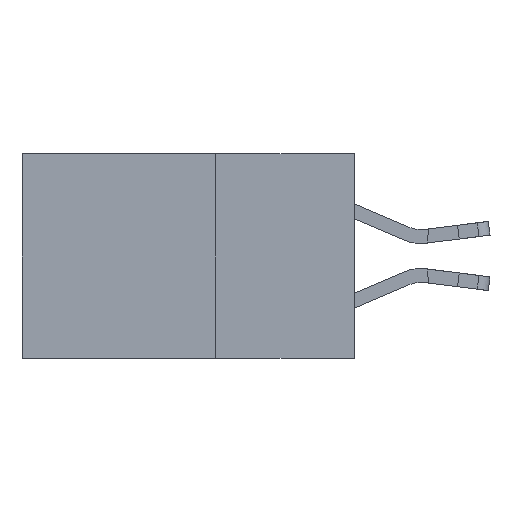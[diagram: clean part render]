
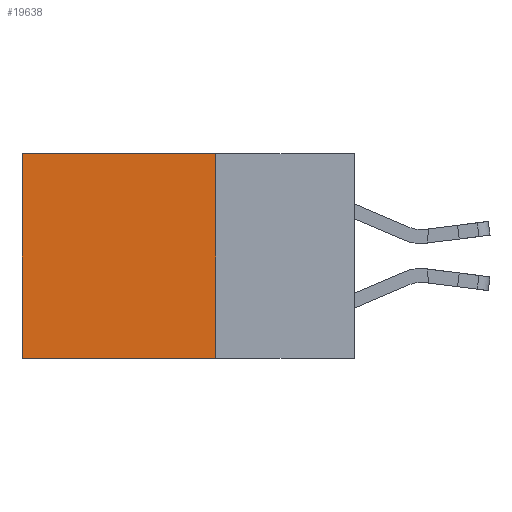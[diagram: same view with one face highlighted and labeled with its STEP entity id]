
A CAD part, left-side view. The second image highlights one B-rep face of the part: STEP entity #19638.
In plain terms, the highlighted planar face has unit normal (-1, 0, 0).
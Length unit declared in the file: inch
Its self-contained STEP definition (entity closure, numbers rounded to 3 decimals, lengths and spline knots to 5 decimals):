
#1786 = LINE ( 'NONE', #7058, #3693 ) ;
#1885 = FACE_OUTER_BOUND ( 'NONE', #11815, .T. ) ;
#1964 = CARTESIAN_POINT ( 'NONE',  ( 0.2615, 0.25, -0.37 ) ) ;
#2830 = VERTEX_POINT ( 'NONE', #12885 ) ;
#3693 = VECTOR ( 'NONE', #8473, 39.37008 ) ;
#6259 = VECTOR ( 'NONE', #14885, 39.37008 ) ;
#6769 = CARTESIAN_POINT ( 'NONE',  ( 0.2615, 0.6, 0. ) ) ;
#7058 = CARTESIAN_POINT ( 'NONE',  ( 0.2615, 0.6, -0.37 ) ) ;
#7278 = PLANE ( 'NONE',  #9597 ) ;
#7681 = CARTESIAN_POINT ( 'NONE',  ( 0.2615, 0.25, 0. ) ) ;
#8473 = DIRECTION ( 'NONE',  ( 0., 0., -1. ) ) ;
#9597 = AXIS2_PLACEMENT_3D ( 'NONE', #12700, #10930, #19912 ) ;
#10844 = ORIENTED_EDGE ( 'NONE', *, *, #21591, .F. ) ;
#10930 = DIRECTION ( 'NONE',  ( 1., 0., 0. ) ) ;
#11192 = ORIENTED_EDGE ( 'NONE', *, *, #12193, .F. ) ;
#11537 = VECTOR ( 'NONE', #14546, 39.37008 ) ;
#11563 = LINE ( 'NONE', #7681, #6259 ) ;
#11815 = EDGE_LOOP ( 'NONE', ( #16681, #10844, #11192, #14252 ) ) ;
#12193 = EDGE_CURVE ( 'NONE', #12238, #22116, #15587, .T. ) ;
#12238 = VERTEX_POINT ( 'NONE', #13575 ) ;
#12433 = LINE ( 'NONE', #1964, #11537 ) ;
#12700 = CARTESIAN_POINT ( 'NONE',  ( 0.2615, 0.25, -0.37 ) ) ;
#12885 = CARTESIAN_POINT ( 'NONE',  ( 0.2615, 0.6, -0.37 ) ) ;
#13575 = CARTESIAN_POINT ( 'NONE',  ( 0.2615, 0.25, 0. ) ) ;
#13687 = CARTESIAN_POINT ( 'NONE',  ( 0.2615, 0.25, -0.37 ) ) ;
#14252 = ORIENTED_EDGE ( 'NONE', *, *, #20661, .T. ) ;
#14546 = DIRECTION ( 'NONE',  ( 0., 1., 0. ) ) ;
#14885 = DIRECTION ( 'NONE',  ( 0., 1., 0. ) ) ;
#15587 = LINE ( 'NONE', #13687, #16256 ) ;
#15950 = CARTESIAN_POINT ( 'NONE',  ( 0.2615, 0.25, -0.37 ) ) ;
#16256 = VECTOR ( 'NONE', #16998, 39.37008 ) ;
#16681 = ORIENTED_EDGE ( 'NONE', *, *, #22537, .T. ) ;
#16998 = DIRECTION ( 'NONE',  ( 0., 0., -1. ) ) ;
#17247 = VERTEX_POINT ( 'NONE', #6769 ) ;
#19638 = ADVANCED_FACE ( 'NONE', ( #1885 ), #7278, .F. ) ;
#19912 = DIRECTION ( 'NONE',  ( 0., 0., -1. ) ) ;
#20661 = EDGE_CURVE ( 'NONE', #12238, #17247, #11563, .T. ) ;
#21591 = EDGE_CURVE ( 'NONE', #22116, #2830, #12433, .T. ) ;
#22116 = VERTEX_POINT ( 'NONE', #15950 ) ;
#22537 = EDGE_CURVE ( 'NONE', #17247, #2830, #1786, .T. ) ;
